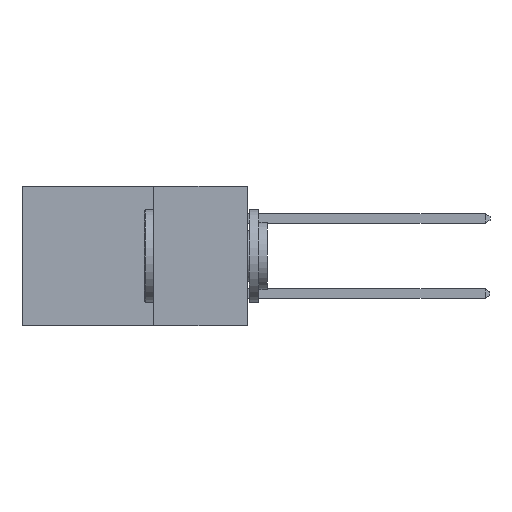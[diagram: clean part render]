
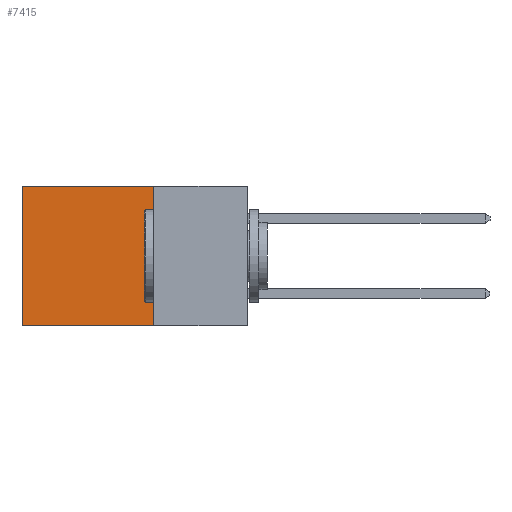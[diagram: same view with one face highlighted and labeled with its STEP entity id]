
A CAD part, left-side view. The second image highlights one B-rep face of the part: STEP entity #7415.
In plain terms, the highlighted planar face has unit normal (-1, 0, 0).
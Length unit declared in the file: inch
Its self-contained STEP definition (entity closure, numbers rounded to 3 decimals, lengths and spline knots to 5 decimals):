
#202 = VECTOR ( 'NONE', #519, 39.37008 ) ;
#519 = DIRECTION ( 'NONE',  ( 0., 1., 0. ) ) ;
#893 = DIRECTION ( 'NONE',  ( 0., 0., -1. ) ) ;
#1530 = CARTESIAN_POINT ( 'NONE',  ( 0.298, 0.25, 0. ) ) ;
#3850 = VECTOR ( 'NONE', #9700, 39.37008 ) ;
#3907 = CARTESIAN_POINT ( 'NONE',  ( 0.298, 0.6, -0.37 ) ) ;
#3972 = VECTOR ( 'NONE', #893, 39.37008 ) ;
#4284 = LINE ( 'NONE', #15844, #202 ) ;
#4473 = LINE ( 'NONE', #1530, #3972 ) ;
#4876 = CARTESIAN_POINT ( 'NONE',  ( 0.298, 0.25, -0.37 ) ) ;
#5072 = CARTESIAN_POINT ( 'NONE',  ( 0.298, 0.6, 0. ) ) ;
#5186 = LINE ( 'NONE', #18014, #12966 ) ;
#5517 = ORIENTED_EDGE ( 'NONE', *, *, #14763, .T. ) ;
#5954 = EDGE_LOOP ( 'NONE', ( #5517, #9744, #6329, #8230 ) ) ;
#6329 = ORIENTED_EDGE ( 'NONE', *, *, #7856, .F. ) ;
#7130 = VERTEX_POINT ( 'NONE', #19188 ) ;
#7415 = ADVANCED_FACE ( 'NONE', ( #7624 ), #11999, .F. ) ;
#7624 = FACE_OUTER_BOUND ( 'NONE', #5954, .T. ) ;
#7856 = EDGE_CURVE ( 'NONE', #10979, #10272, #4473, .T. ) ;
#8230 = ORIENTED_EDGE ( 'NONE', *, *, #11651, .T. ) ;
#9700 = DIRECTION ( 'NONE',  ( 0., 0., -1. ) ) ;
#9744 = ORIENTED_EDGE ( 'NONE', *, *, #16019, .F. ) ;
#10272 = VERTEX_POINT ( 'NONE', #4876 ) ;
#10979 = VERTEX_POINT ( 'NONE', #15698 ) ;
#11651 = EDGE_CURVE ( 'NONE', #10979, #7130, #5186, .T. ) ;
#11867 = DIRECTION ( 'NONE',  ( 0., 0., -1. ) ) ;
#11870 = DIRECTION ( 'NONE',  ( 1., 0., 0. ) ) ;
#11928 = CARTESIAN_POINT ( 'NONE',  ( 0.298, 0.25, 0. ) ) ;
#11999 = PLANE ( 'NONE',  #17262 ) ;
#12966 = VECTOR ( 'NONE', #17997, 39.37008 ) ;
#13441 = VERTEX_POINT ( 'NONE', #3907 ) ;
#14763 = EDGE_CURVE ( 'NONE', #7130, #13441, #16561, .T. ) ;
#15698 = CARTESIAN_POINT ( 'NONE',  ( 0.298, 0.25, 0. ) ) ;
#15844 = CARTESIAN_POINT ( 'NONE',  ( 0.298, 0.25, -0.37 ) ) ;
#16019 = EDGE_CURVE ( 'NONE', #10272, #13441, #4284, .T. ) ;
#16561 = LINE ( 'NONE', #5072, #3850 ) ;
#17262 = AXIS2_PLACEMENT_3D ( 'NONE', #11928, #11870, #11867 ) ;
#17997 = DIRECTION ( 'NONE',  ( 0., 1., 0. ) ) ;
#18014 = CARTESIAN_POINT ( 'NONE',  ( 0.298, 0.25, 0. ) ) ;
#19188 = CARTESIAN_POINT ( 'NONE',  ( 0.298, 0.6, 0. ) ) ;
